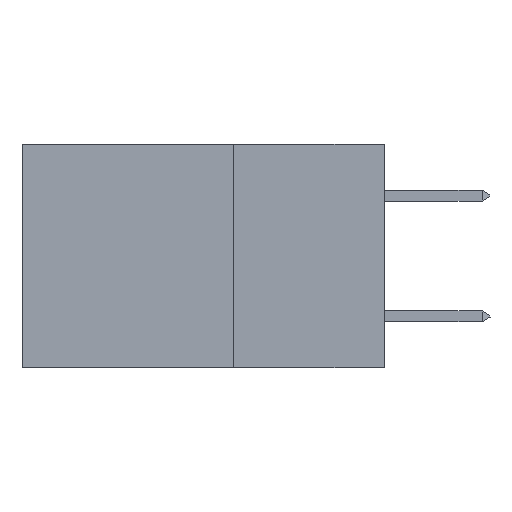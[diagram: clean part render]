
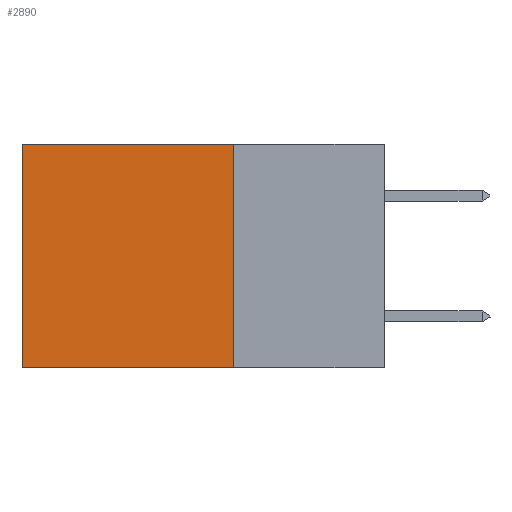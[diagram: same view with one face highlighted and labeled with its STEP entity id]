
A CAD part, left-side view. The second image highlights one B-rep face of the part: STEP entity #2890.
In plain terms, the highlighted planar face has unit normal (-1, 0, 0).
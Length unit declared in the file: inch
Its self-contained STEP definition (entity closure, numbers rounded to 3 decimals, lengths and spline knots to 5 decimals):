
#338 = LINE ( 'NONE', #4162, #8335 ) ;
#396 = DIRECTION ( 'NONE',  ( 1., 0., 0. ) ) ;
#1344 = ORIENTED_EDGE ( 'NONE', *, *, #14165, .F. ) ;
#1356 = CARTESIAN_POINT ( 'NONE',  ( 0.2875, 0.25, 0. ) ) ;
#2329 = AXIS2_PLACEMENT_3D ( 'NONE', #10858, #396, #2432 ) ;
#2432 = DIRECTION ( 'NONE',  ( 0., 0., -1. ) ) ;
#2890 = ADVANCED_FACE ( 'NONE', ( #18649 ), #8188, .F. ) ;
#2942 = VERTEX_POINT ( 'NONE', #10067 ) ;
#3876 = ORIENTED_EDGE ( 'NONE', *, *, #18227, .F. ) ;
#4162 = CARTESIAN_POINT ( 'NONE',  ( 0.2875, 0.25, -0.37 ) ) ;
#4411 = LINE ( 'NONE', #1356, #13053 ) ;
#5731 = DIRECTION ( 'NONE',  ( 0., 1., 0. ) ) ;
#5847 = DIRECTION ( 'NONE',  ( 0., 0., -1. ) ) ;
#6149 = DIRECTION ( 'NONE',  ( 0., 1., 0. ) ) ;
#6892 = ORIENTED_EDGE ( 'NONE', *, *, #16658, .T. ) ;
#7542 = VECTOR ( 'NONE', #11282, 39.37008 ) ;
#8181 = VERTEX_POINT ( 'NONE', #15879 ) ;
#8188 = PLANE ( 'NONE',  #2329 ) ;
#8335 = VECTOR ( 'NONE', #5731, 39.37008 ) ;
#8564 = CARTESIAN_POINT ( 'NONE',  ( 0.2875, 0.25, 0. ) ) ;
#9260 = VECTOR ( 'NONE', #5847, 39.37008 ) ;
#9605 = CARTESIAN_POINT ( 'NONE',  ( 0.2875, 0.6, -0.37 ) ) ;
#9706 = LINE ( 'NONE', #17610, #9260 ) ;
#9742 = CARTESIAN_POINT ( 'NONE',  ( 0.2875, 0.25, 0. ) ) ;
#10067 = CARTESIAN_POINT ( 'NONE',  ( 0.2875, 0.6, 0. ) ) ;
#10858 = CARTESIAN_POINT ( 'NONE',  ( 0.2875, 0.25, 0. ) ) ;
#11282 = DIRECTION ( 'NONE',  ( 0., 0., -1. ) ) ;
#11544 = LINE ( 'NONE', #9742, #7542 ) ;
#12240 = VERTEX_POINT ( 'NONE', #8564 ) ;
#12838 = EDGE_LOOP ( 'NONE', ( #6892, #1344, #3876, #17284 ) ) ;
#13053 = VECTOR ( 'NONE', #6149, 39.37008 ) ;
#13732 = EDGE_CURVE ( 'NONE', #12240, #2942, #4411, .T. ) ;
#14165 = EDGE_CURVE ( 'NONE', #8181, #15164, #338, .T. ) ;
#15164 = VERTEX_POINT ( 'NONE', #9605 ) ;
#15879 = CARTESIAN_POINT ( 'NONE',  ( 0.2875, 0.25, -0.37 ) ) ;
#16658 = EDGE_CURVE ( 'NONE', #2942, #15164, #9706, .T. ) ;
#17284 = ORIENTED_EDGE ( 'NONE', *, *, #13732, .T. ) ;
#17610 = CARTESIAN_POINT ( 'NONE',  ( 0.2875, 0.6, 0. ) ) ;
#18227 = EDGE_CURVE ( 'NONE', #12240, #8181, #11544, .T. ) ;
#18649 = FACE_OUTER_BOUND ( 'NONE', #12838, .T. ) ;
